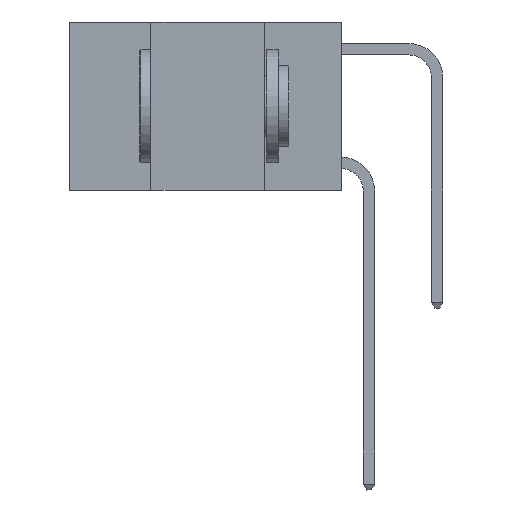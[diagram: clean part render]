
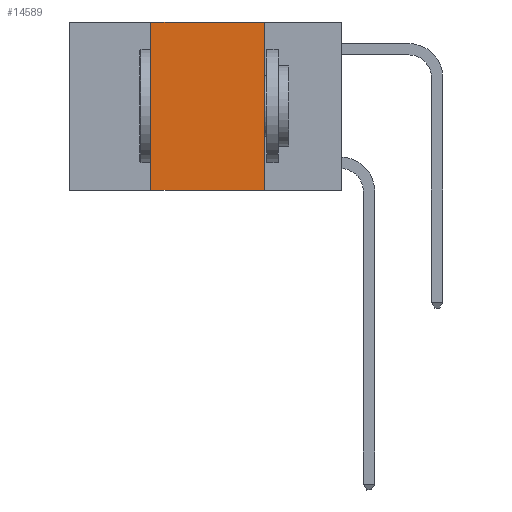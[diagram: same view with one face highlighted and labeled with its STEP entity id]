
A CAD part, left-side view. The second image highlights one B-rep face of the part: STEP entity #14589.
In plain terms, the highlighted planar face has unit normal (-1, 0, 0).
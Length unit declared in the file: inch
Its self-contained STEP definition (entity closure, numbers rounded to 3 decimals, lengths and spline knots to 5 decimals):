
#481 = CARTESIAN_POINT ( 'NONE',  ( 0., 0.6, -0.37 ) ) ;
#766 = LINE ( 'NONE', #481, #3365 ) ;
#2142 = VERTEX_POINT ( 'NONE', #3793 ) ;
#3230 = ORIENTED_EDGE ( 'NONE', *, *, #19467, .F. ) ;
#3365 = VECTOR ( 'NONE', #7007, 39.37008 ) ;
#3600 = LINE ( 'NONE', #8485, #5713 ) ;
#3793 = CARTESIAN_POINT ( 'NONE',  ( 0., 0.42, -0.37 ) ) ;
#3808 = ORIENTED_EDGE ( 'NONE', *, *, #8798, .F. ) ;
#3997 = VECTOR ( 'NONE', #12371, 39.37008 ) ;
#4253 = VECTOR ( 'NONE', #13557, 39.37008 ) ;
#5019 = DIRECTION ( 'NONE',  ( 0., 0., 1. ) ) ;
#5066 = CARTESIAN_POINT ( 'NONE',  ( 0., 0.6, 0. ) ) ;
#5713 = VECTOR ( 'NONE', #5019, 39.37008 ) ;
#6547 = EDGE_CURVE ( 'NONE', #2142, #6730, #766, .T. ) ;
#6689 = CARTESIAN_POINT ( 'NONE',  ( 0., 0.42, 0. ) ) ;
#6730 = VERTEX_POINT ( 'NONE', #9036 ) ;
#6776 = VERTEX_POINT ( 'NONE', #8931 ) ;
#6803 = EDGE_CURVE ( 'NONE', #8344, #6776, #15402, .T. ) ;
#7007 = DIRECTION ( 'NONE',  ( 0., -1., 0. ) ) ;
#7144 = EDGE_LOOP ( 'NONE', ( #3230, #16126, #3808, #9534 ) ) ;
#8243 = DIRECTION ( 'NONE',  ( 0., 0., -1. ) ) ;
#8344 = VERTEX_POINT ( 'NONE', #6689 ) ;
#8485 = CARTESIAN_POINT ( 'NONE',  ( 0., 0.42, 0. ) ) ;
#8798 = EDGE_CURVE ( 'NONE', #2142, #8344, #3600, .T. ) ;
#8931 = CARTESIAN_POINT ( 'NONE',  ( 0., 0.17, 0. ) ) ;
#9036 = CARTESIAN_POINT ( 'NONE',  ( 0., 0.17, -0.37 ) ) ;
#9534 = ORIENTED_EDGE ( 'NONE', *, *, #6547, .T. ) ;
#12371 = DIRECTION ( 'NONE',  ( 0., -1., 0. ) ) ;
#13277 = AXIS2_PLACEMENT_3D ( 'NONE', #5066, #17648, #8243 ) ;
#13557 = DIRECTION ( 'NONE',  ( 0., 0., -1. ) ) ;
#13837 = PLANE ( 'NONE',  #13277 ) ;
#13970 = LINE ( 'NONE', #18218, #4253 ) ;
#14589 = ADVANCED_FACE ( 'NONE', ( #15336 ), #13837, .F. ) ;
#15336 = FACE_OUTER_BOUND ( 'NONE', #7144, .T. ) ;
#15402 = LINE ( 'NONE', #16815, #3997 ) ;
#16126 = ORIENTED_EDGE ( 'NONE', *, *, #6803, .F. ) ;
#16815 = CARTESIAN_POINT ( 'NONE',  ( 0., 0.6, 0. ) ) ;
#17648 = DIRECTION ( 'NONE',  ( 1., 0., 0. ) ) ;
#18218 = CARTESIAN_POINT ( 'NONE',  ( 0., 0.17, 0. ) ) ;
#19467 = EDGE_CURVE ( 'NONE', #6776, #6730, #13970, .T. ) ;
